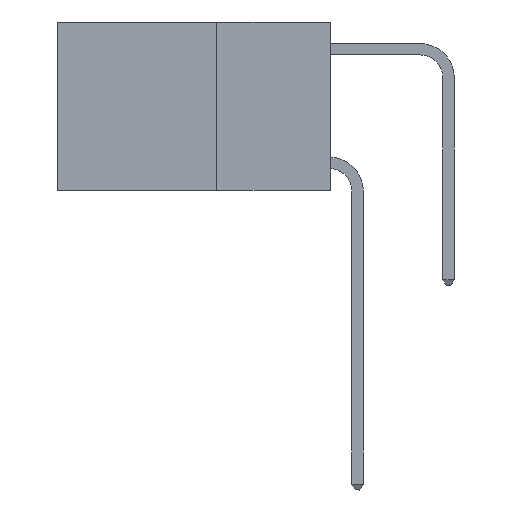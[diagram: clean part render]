
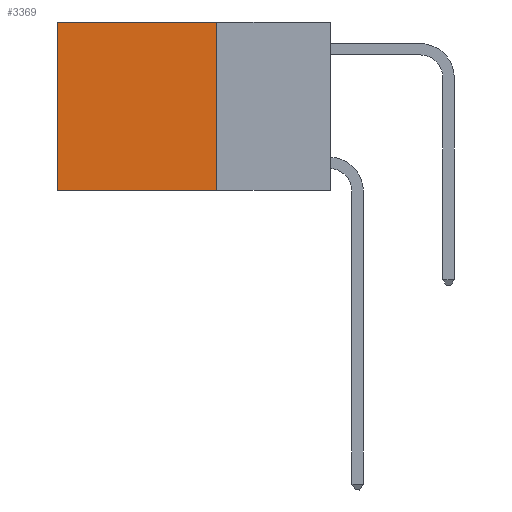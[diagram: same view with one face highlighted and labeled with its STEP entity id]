
A CAD part, left-side view. The second image highlights one B-rep face of the part: STEP entity #3369.
In plain terms, the highlighted planar face has unit normal (-1, 0, 0).
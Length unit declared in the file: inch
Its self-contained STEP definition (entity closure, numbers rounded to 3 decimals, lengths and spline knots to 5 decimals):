
#1164 = DIRECTION ( 'NONE',  ( 1., 0., 0. ) ) ;
#2406 = DIRECTION ( 'NONE',  ( 0., 0., -1. ) ) ;
#2676 = VERTEX_POINT ( 'NONE', #4181 ) ;
#3155 = PLANE ( 'NONE',  #19305 ) ;
#3221 = CARTESIAN_POINT ( 'NONE',  ( 0.2625, 0.25, 0. ) ) ;
#3369 = ADVANCED_FACE ( 'NONE', ( #19646 ), #3155, .F. ) ;
#4181 = CARTESIAN_POINT ( 'NONE',  ( 0.2625, 0.6, 0. ) ) ;
#4470 = LINE ( 'NONE', #3221, #22370 ) ;
#4587 = DIRECTION ( 'NONE',  ( 0., 0., -1. ) ) ;
#7384 = EDGE_CURVE ( 'NONE', #23708, #2676, #4470, .T. ) ;
#7689 = CARTESIAN_POINT ( 'NONE',  ( 0.2625, 0.25, 0. ) ) ;
#8130 = CARTESIAN_POINT ( 'NONE',  ( 0.2625, 0.25, 0. ) ) ;
#9281 = DIRECTION ( 'NONE',  ( 0., 0., -1. ) ) ;
#9966 = VECTOR ( 'NONE', #2406, 39.37008 ) ;
#11266 = CARTESIAN_POINT ( 'NONE',  ( 0.2625, 0.25, 0. ) ) ;
#11618 = ORIENTED_EDGE ( 'NONE', *, *, #18502, .F. ) ;
#12392 = CARTESIAN_POINT ( 'NONE',  ( 0.2625, 0.6, -0.37 ) ) ;
#14502 = CARTESIAN_POINT ( 'NONE',  ( 0.2625, 0.25, -0.37 ) ) ;
#14933 = CARTESIAN_POINT ( 'NONE',  ( 0.2625, 0.25, -0.37 ) ) ;
#15337 = LINE ( 'NONE', #14933, #22704 ) ;
#16691 = DIRECTION ( 'NONE',  ( 0., 1., 0. ) ) ;
#16752 = LINE ( 'NONE', #8130, #9966 ) ;
#16897 = EDGE_CURVE ( 'NONE', #2676, #17302, #18549, .T. ) ;
#17302 = VERTEX_POINT ( 'NONE', #12392 ) ;
#17362 = ORIENTED_EDGE ( 'NONE', *, *, #16897, .T. ) ;
#17659 = ORIENTED_EDGE ( 'NONE', *, *, #20382, .F. ) ;
#18502 = EDGE_CURVE ( 'NONE', #21779, #17302, #15337, .T. ) ;
#18549 = LINE ( 'NONE', #22805, #21805 ) ;
#19245 = EDGE_LOOP ( 'NONE', ( #17362, #11618, #17659, #20433 ) ) ;
#19305 = AXIS2_PLACEMENT_3D ( 'NONE', #11266, #1164, #9281 ) ;
#19646 = FACE_OUTER_BOUND ( 'NONE', #19245, .T. ) ;
#20382 = EDGE_CURVE ( 'NONE', #23708, #21779, #16752, .T. ) ;
#20433 = ORIENTED_EDGE ( 'NONE', *, *, #7384, .T. ) ;
#20909 = DIRECTION ( 'NONE',  ( 0., 1., 0. ) ) ;
#21779 = VERTEX_POINT ( 'NONE', #14502 ) ;
#21805 = VECTOR ( 'NONE', #4587, 39.37008 ) ;
#22370 = VECTOR ( 'NONE', #16691, 39.37008 ) ;
#22704 = VECTOR ( 'NONE', #20909, 39.37008 ) ;
#22805 = CARTESIAN_POINT ( 'NONE',  ( 0.2625, 0.6, 0. ) ) ;
#23708 = VERTEX_POINT ( 'NONE', #7689 ) ;
